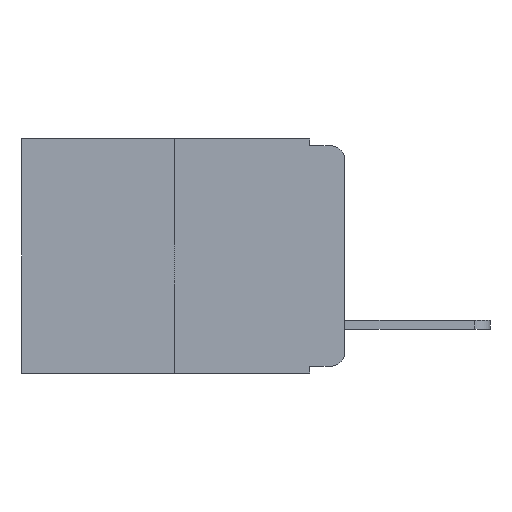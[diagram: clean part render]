
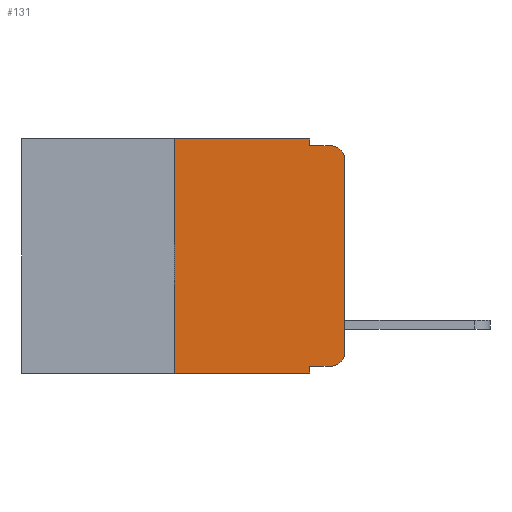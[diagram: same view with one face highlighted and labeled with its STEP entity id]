
A CAD part, left-side view. The second image highlights one B-rep face of the part: STEP entity #131.
In plain terms, the highlighted planar face has unit normal (-1, 0, 0).
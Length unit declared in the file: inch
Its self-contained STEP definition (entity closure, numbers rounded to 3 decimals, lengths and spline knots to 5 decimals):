
#131 = ADVANCED_FACE ( 'NONE', ( #12965 ), #8603, .F. ) ;
#462 = VERTEX_POINT ( 'NONE', #12632 ) ;
#715 = CARTESIAN_POINT ( 'NONE',  ( 0., 0.02, -0.333 ) ) ;
#1018 = AXIS2_PLACEMENT_3D ( 'NONE', #16927, #7823, #18276 ) ;
#1155 = ORIENTED_EDGE ( 'NONE', *, *, #12624, .T. ) ;
#1196 = VERTEX_POINT ( 'NONE', #19771 ) ;
#1511 = VERTEX_POINT ( 'NONE', #19220 ) ;
#2024 = ORIENTED_EDGE ( 'NONE', *, *, #13037, .T. ) ;
#2031 = CARTESIAN_POINT ( 'NONE',  ( 0., 0.02, -0.03 ) ) ;
#2666 = CARTESIAN_POINT ( 'NONE',  ( 0., 0.473, 0. ) ) ;
#3860 = DIRECTION ( 'NONE',  ( 0., 0., -1. ) ) ;
#3931 = CARTESIAN_POINT ( 'NONE',  ( 0., 0.473, 0. ) ) ;
#4027 = DIRECTION ( 'NONE',  ( 0., 0., -1. ) ) ;
#4369 = LINE ( 'NONE', #16641, #9286 ) ;
#4386 = VERTEX_POINT ( 'NONE', #15056 ) ;
#4437 = VECTOR ( 'NONE', #16948, 39.37008 ) ;
#4805 = ORIENTED_EDGE ( 'NONE', *, *, #12471, .F. ) ;
#5481 = CARTESIAN_POINT ( 'NONE',  ( 0., 0.051, -0.333 ) ) ;
#5568 = AXIS2_PLACEMENT_3D ( 'NONE', #2031, #13631, #3860 ) ;
#5998 = LINE ( 'NONE', #7320, #9775 ) ;
#6089 = CARTESIAN_POINT ( 'NONE',  ( 0., 0.051, 0. ) ) ;
#6159 = VERTEX_POINT ( 'NONE', #5481 ) ;
#6473 = VERTEX_POINT ( 'NONE', #7802 ) ;
#6488 = CIRCLE ( 'NONE', #1018, 0.02 ) ;
#6522 = CIRCLE ( 'NONE', #5568, 0.02 ) ;
#6917 = ORIENTED_EDGE ( 'NONE', *, *, #12508, .F. ) ;
#7222 = ORIENTED_EDGE ( 'NONE', *, *, #11726, .T. ) ;
#7320 = CARTESIAN_POINT ( 'NONE',  ( 0., 0.051, -0.01 ) ) ;
#7650 = ORIENTED_EDGE ( 'NONE', *, *, #12416, .F. ) ;
#7713 = DIRECTION ( 'NONE',  ( 0., 0., -1. ) ) ;
#7797 = CARTESIAN_POINT ( 'NONE',  ( 0., 0.051, -0.343 ) ) ;
#7802 = CARTESIAN_POINT ( 'NONE',  ( 0., 0.051, 0. ) ) ;
#7823 = DIRECTION ( 'NONE',  ( -1., 0., 0. ) ) ;
#7974 = DIRECTION ( 'NONE',  ( 0., -1., 0. ) ) ;
#8218 = VERTEX_POINT ( 'NONE', #12077 ) ;
#8325 = DIRECTION ( 'NONE',  ( 1., 0., 0. ) ) ;
#8416 = CARTESIAN_POINT ( 'NONE',  ( 0., 0., 0. ) ) ;
#8603 = PLANE ( 'NONE',  #19306 ) ;
#8824 = LINE ( 'NONE', #2666, #4437 ) ;
#9286 = VECTOR ( 'NONE', #4027, 39.37008 ) ;
#9660 = ORIENTED_EDGE ( 'NONE', *, *, #10971, .F. ) ;
#9775 = VECTOR ( 'NONE', #15136, 39.37008 ) ;
#9925 = EDGE_LOOP ( 'NONE', ( #14733, #18597, #7650, #4805, #9660, #6917, #7222, #17196, #1155, #2024 ) ) ;
#10022 = VECTOR ( 'NONE', #10024, 39.37008 ) ;
#10024 = DIRECTION ( 'NONE',  ( 0., 0., 1. ) ) ;
#10971 = EDGE_CURVE ( 'NONE', #462, #6473, #8824, .T. ) ;
#11504 = CARTESIAN_POINT ( 'NONE',  ( 0., 0.473, -0.343 ) ) ;
#11726 = EDGE_CURVE ( 'NONE', #1511, #13552, #12015, .T. ) ;
#12015 = LINE ( 'NONE', #11504, #19113 ) ;
#12077 = CARTESIAN_POINT ( 'NONE',  ( 0., 0.051, -0.01 ) ) ;
#12254 = EDGE_CURVE ( 'NONE', #1196, #19793, #17897, .T. ) ;
#12383 = EDGE_CURVE ( 'NONE', #19793, #4386, #6522, .T. ) ;
#12416 = EDGE_CURVE ( 'NONE', #8218, #4386, #5998, .T. ) ;
#12471 = EDGE_CURVE ( 'NONE', #6473, #8218, #4369, .T. ) ;
#12508 = EDGE_CURVE ( 'NONE', #1511, #462, #15508, .T. ) ;
#12531 = EDGE_CURVE ( 'NONE', #6159, #13552, #15073, .T. ) ;
#12624 = EDGE_CURVE ( 'NONE', #6159, #17485, #16575, .T. ) ;
#12632 = CARTESIAN_POINT ( 'NONE',  ( 0., 0.25, 0. ) ) ;
#12965 = FACE_OUTER_BOUND ( 'NONE', #9925, .T. ) ;
#13037 = EDGE_CURVE ( 'NONE', #17485, #1196, #6488, .T. ) ;
#13552 = VERTEX_POINT ( 'NONE', #7797 ) ;
#13631 = DIRECTION ( 'NONE',  ( -1., 0., 0. ) ) ;
#14733 = ORIENTED_EDGE ( 'NONE', *, *, #12254, .T. ) ;
#15056 = CARTESIAN_POINT ( 'NONE',  ( 0., 0.02, -0.01 ) ) ;
#15073 = LINE ( 'NONE', #6089, #18695 ) ;
#15136 = DIRECTION ( 'NONE',  ( 0., -1., 0. ) ) ;
#15380 = CARTESIAN_POINT ( 'NONE',  ( 0., 0.25, 0. ) ) ;
#15508 = LINE ( 'NONE', #15380, #16362 ) ;
#16362 = VECTOR ( 'NONE', #19437, 39.37008 ) ;
#16575 = LINE ( 'NONE', #18410, #17016 ) ;
#16641 = CARTESIAN_POINT ( 'NONE',  ( 0., 0.051, 0. ) ) ;
#16927 = CARTESIAN_POINT ( 'NONE',  ( 0., 0.02, -0.313 ) ) ;
#16948 = DIRECTION ( 'NONE',  ( 0., -1., 0. ) ) ;
#17016 = VECTOR ( 'NONE', #7974, 39.37008 ) ;
#17072 = DIRECTION ( 'NONE',  ( 0., 0., -1. ) ) ;
#17196 = ORIENTED_EDGE ( 'NONE', *, *, #12531, .F. ) ;
#17485 = VERTEX_POINT ( 'NONE', #715 ) ;
#17897 = LINE ( 'NONE', #8416, #10022 ) ;
#18276 = DIRECTION ( 'NONE',  ( 0., 0., -1. ) ) ;
#18410 = CARTESIAN_POINT ( 'NONE',  ( 0., 0.051, -0.333 ) ) ;
#18597 = ORIENTED_EDGE ( 'NONE', *, *, #12383, .T. ) ;
#18695 = VECTOR ( 'NONE', #7713, 39.37008 ) ;
#19029 = CARTESIAN_POINT ( 'NONE',  ( 0., 0., -0.03 ) ) ;
#19113 = VECTOR ( 'NONE', #20049, 39.37008 ) ;
#19220 = CARTESIAN_POINT ( 'NONE',  ( 0., 0.25, -0.343 ) ) ;
#19306 = AXIS2_PLACEMENT_3D ( 'NONE', #3931, #8325, #17072 ) ;
#19437 = DIRECTION ( 'NONE',  ( 0., 0., 1. ) ) ;
#19771 = CARTESIAN_POINT ( 'NONE',  ( 0., 0., -0.313 ) ) ;
#19793 = VERTEX_POINT ( 'NONE', #19029 ) ;
#20049 = DIRECTION ( 'NONE',  ( 0., -1., 0. ) ) ;
